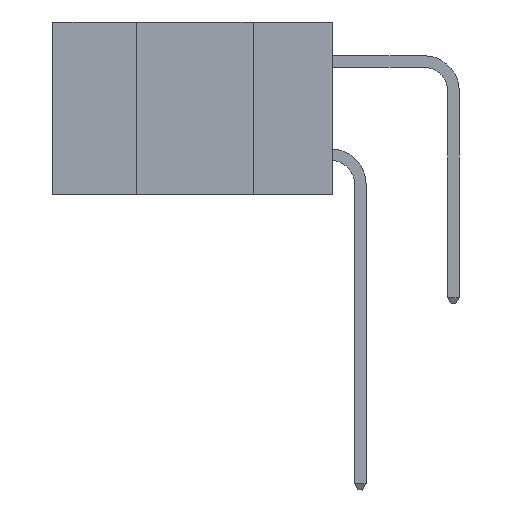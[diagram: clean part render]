
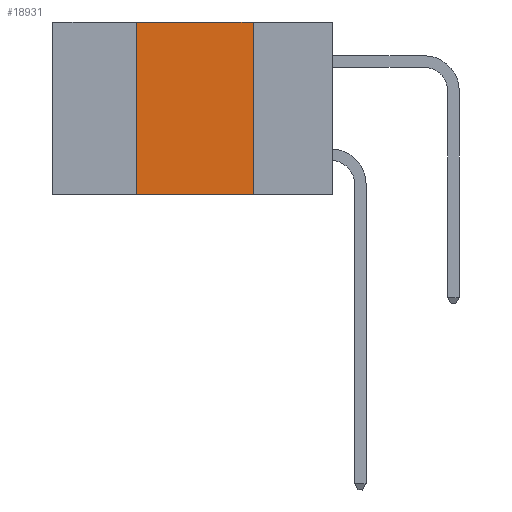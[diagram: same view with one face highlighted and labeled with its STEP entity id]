
A CAD part, left-side view. The second image highlights one B-rep face of the part: STEP entity #18931.
In plain terms, the highlighted planar face has unit normal (-1, 0, 0).
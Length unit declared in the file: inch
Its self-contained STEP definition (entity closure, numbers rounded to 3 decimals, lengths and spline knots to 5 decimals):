
#1840 = VECTOR ( 'NONE', #13708, 39.37008 ) ;
#1897 = PLANE ( 'NONE',  #8312 ) ;
#3107 = ORIENTED_EDGE ( 'NONE', *, *, #17390, .F. ) ;
#3966 = VERTEX_POINT ( 'NONE', #34840 ) ;
#4334 = CARTESIAN_POINT ( 'NONE',  ( 0., 0.17, 0. ) ) ;
#5491 = VECTOR ( 'NONE', #26556, 39.37008 ) ;
#5998 = ORIENTED_EDGE ( 'NONE', *, *, #11074, .T. ) ;
#7529 = EDGE_CURVE ( 'NONE', #3966, #34127, #9330, .T. ) ;
#8312 = AXIS2_PLACEMENT_3D ( 'NONE', #20889, #21120, #13188 ) ;
#9330 = LINE ( 'NONE', #15296, #5491 ) ;
#9469 = LINE ( 'NONE', #29940, #1840 ) ;
#11074 = EDGE_CURVE ( 'NONE', #3966, #23264, #9469, .T. ) ;
#11410 = VECTOR ( 'NONE', #12683, 39.37008 ) ;
#12683 = DIRECTION ( 'NONE',  ( 0., 0., -1. ) ) ;
#13188 = DIRECTION ( 'NONE',  ( 0., 0., -1. ) ) ;
#13708 = DIRECTION ( 'NONE',  ( 0., -1., 0. ) ) ;
#15296 = CARTESIAN_POINT ( 'NONE',  ( 0., 0.42, 0. ) ) ;
#15327 = LINE ( 'NONE', #20370, #25088 ) ;
#16588 = CARTESIAN_POINT ( 'NONE',  ( 0., 0.42, 0. ) ) ;
#17250 = VERTEX_POINT ( 'NONE', #22617 ) ;
#17390 = EDGE_CURVE ( 'NONE', #34127, #17250, #15327, .T. ) ;
#18931 = ADVANCED_FACE ( 'NONE', ( #23780 ), #1897, .F. ) ;
#19543 = EDGE_CURVE ( 'NONE', #17250, #23264, #34826, .T. ) ;
#20370 = CARTESIAN_POINT ( 'NONE',  ( 0., 0.6, 0. ) ) ;
#20889 = CARTESIAN_POINT ( 'NONE',  ( 0., 0.6, 0. ) ) ;
#21120 = DIRECTION ( 'NONE',  ( 1., 0., 0. ) ) ;
#22617 = CARTESIAN_POINT ( 'NONE',  ( 0., 0.17, 0. ) ) ;
#23264 = VERTEX_POINT ( 'NONE', #25881 ) ;
#23441 = DIRECTION ( 'NONE',  ( 0., -1., 0. ) ) ;
#23780 = FACE_OUTER_BOUND ( 'NONE', #24996, .T. ) ;
#24996 = EDGE_LOOP ( 'NONE', ( #26675, #3107, #25515, #5998 ) ) ;
#25088 = VECTOR ( 'NONE', #23441, 39.37008 ) ;
#25515 = ORIENTED_EDGE ( 'NONE', *, *, #7529, .F. ) ;
#25881 = CARTESIAN_POINT ( 'NONE',  ( 0., 0.17, -0.37 ) ) ;
#26556 = DIRECTION ( 'NONE',  ( 0., 0., 1. ) ) ;
#26675 = ORIENTED_EDGE ( 'NONE', *, *, #19543, .F. ) ;
#29940 = CARTESIAN_POINT ( 'NONE',  ( 0., 0.6, -0.37 ) ) ;
#34127 = VERTEX_POINT ( 'NONE', #16588 ) ;
#34826 = LINE ( 'NONE', #4334, #11410 ) ;
#34840 = CARTESIAN_POINT ( 'NONE',  ( 0., 0.42, -0.37 ) ) ;
